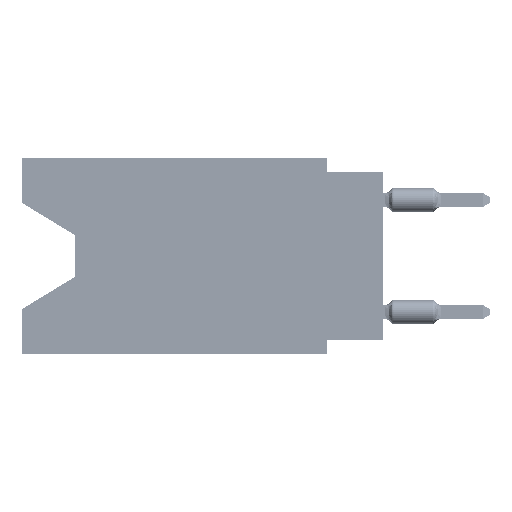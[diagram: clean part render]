
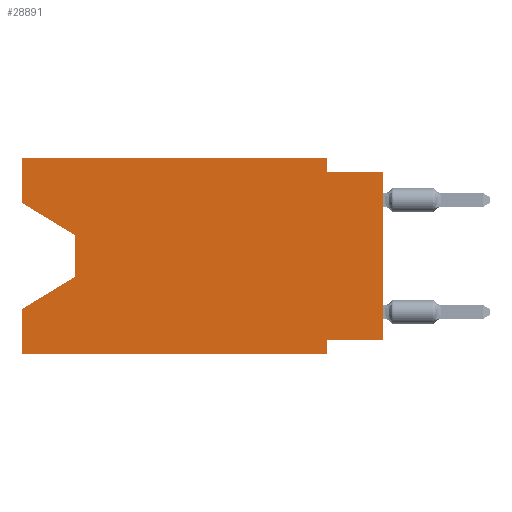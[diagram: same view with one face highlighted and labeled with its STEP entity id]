
A CAD part, left-side view. The second image highlights one B-rep face of the part: STEP entity #28891.
In plain terms, the highlighted planar face has unit normal (-1, 0, 0).
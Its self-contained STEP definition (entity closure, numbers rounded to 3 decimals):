
#560 = CARTESIAN_POINT ( 'NONE',  ( 0., 16.383, -6.852 ) ) ;
#1121 = ORIENTED_EDGE ( 'NONE', *, *, #41987, .T. ) ;
#3770 = VECTOR ( 'NONE', #63906, 1000. ) ;
#4355 = DIRECTION ( 'NONE',  ( 0., 1., 0. ) ) ;
#5054 = ORIENTED_EDGE ( 'NONE', *, *, #59475, .F. ) ;
#6071 = ORIENTED_EDGE ( 'NONE', *, *, #56471, .T. ) ;
#8778 = ORIENTED_EDGE ( 'NONE', *, *, #46111, .F. ) ;
#10045 = EDGE_CURVE ( 'NONE', #20409, #16009, #28303, .T. ) ;
#10096 = DIRECTION ( 'NONE',  ( 0., -1., 0. ) ) ;
#10343 = VECTOR ( 'NONE', #23110, 1000. ) ;
#10506 = ORIENTED_EDGE ( 'NONE', *, *, #18751, .T. ) ;
#11762 = VECTOR ( 'NONE', #4355, 1000. ) ;
#12016 = CARTESIAN_POINT ( 'NONE',  ( 0., 0., -8.255 ) ) ;
#12068 = CARTESIAN_POINT ( 'NONE',  ( 0., 16.383, -2.038 ) ) ;
#12527 = VERTEX_POINT ( 'NONE', #19864 ) ;
#12535 = CARTESIAN_POINT ( 'NONE',  ( 0., 16.383, -2.038 ) ) ;
#14194 = EDGE_CURVE ( 'NONE', #54865, #21545, #33069, .T. ) ;
#14480 = DIRECTION ( 'NONE',  ( 0., 0., 1. ) ) ;
#14519 = EDGE_CURVE ( 'NONE', #12527, #45243, #57657, .T. ) ;
#15418 = LINE ( 'NONE', #22644, #11762 ) ;
#16009 = VERTEX_POINT ( 'NONE', #64974 ) ;
#16568 = PLANE ( 'NONE',  #68132 ) ;
#17599 = DIRECTION ( 'NONE',  ( 0., 0., 1. ) ) ;
#18534 = CARTESIAN_POINT ( 'NONE',  ( 0., 16.383, 0. ) ) ;
#18751 = EDGE_CURVE ( 'NONE', #20409, #54865, #30435, .T. ) ;
#19864 = CARTESIAN_POINT ( 'NONE',  ( 0., 2.54, -0.635 ) ) ;
#20268 = CARTESIAN_POINT ( 'NONE',  ( 0., 16.383, -8.89 ) ) ;
#20409 = VERTEX_POINT ( 'NONE', #12068 ) ;
#21099 = VERTEX_POINT ( 'NONE', #33306 ) ;
#21545 = VERTEX_POINT ( 'NONE', #29250 ) ;
#21775 = ORIENTED_EDGE ( 'NONE', *, *, #10045, .F. ) ;
#22197 = DIRECTION ( 'NONE',  ( 0., -1., 0. ) ) ;
#22376 = CARTESIAN_POINT ( 'NONE',  ( 0., 13.97, -3.505 ) ) ;
#22507 = CARTESIAN_POINT ( 'NONE',  ( 0., 2.54, -8.89 ) ) ;
#22644 = CARTESIAN_POINT ( 'NONE',  ( 0., 0., -8.255 ) ) ;
#22863 = VECTOR ( 'NONE', #27706, 1000. ) ;
#23110 = DIRECTION ( 'NONE',  ( 0., 0., 1. ) ) ;
#23368 = DIRECTION ( 'NONE',  ( 0., 0.855, -0.519 ) ) ;
#24882 = LINE ( 'NONE', #20268, #63633 ) ;
#26849 = CARTESIAN_POINT ( 'NONE',  ( 0., 16.383, 0. ) ) ;
#27547 = CARTESIAN_POINT ( 'NONE',  ( 0., 16.383, -8.89 ) ) ;
#27696 = LINE ( 'NONE', #46357, #3770 ) ;
#27706 = DIRECTION ( 'NONE',  ( 0., 0., -1. ) ) ;
#28303 = LINE ( 'NONE', #29426, #34003 ) ;
#28891 = ADVANCED_FACE ( 'NONE', ( #69191 ), #16568, .F. ) ;
#29250 = CARTESIAN_POINT ( 'NONE',  ( 0., 13.97, -5.385 ) ) ;
#29426 = CARTESIAN_POINT ( 'NONE',  ( 0., 16.383, 0. ) ) ;
#30435 = LINE ( 'NONE', #12535, #47623 ) ;
#31227 = EDGE_CURVE ( 'NONE', #48847, #12527, #27696, .T. ) ;
#31349 = DIRECTION ( 'NONE',  ( 0., -1., 0. ) ) ;
#32784 = CARTESIAN_POINT ( 'NONE',  ( 0., 0., -0.635 ) ) ;
#33069 = LINE ( 'NONE', #22376, #22863 ) ;
#33306 = CARTESIAN_POINT ( 'NONE',  ( 0., 2.54, -8.89 ) ) ;
#33958 = ORIENTED_EDGE ( 'NONE', *, *, #34005, .T. ) ;
#34003 = VECTOR ( 'NONE', #17599, 1000. ) ;
#34005 = EDGE_CURVE ( 'NONE', #21545, #65468, #58437, .T. ) ;
#37012 = CARTESIAN_POINT ( 'NONE',  ( 0., 0., 0. ) ) ;
#38699 = DIRECTION ( 'NONE',  ( 0., 0., -1. ) ) ;
#41537 = VECTOR ( 'NONE', #69793, 1000. ) ;
#41711 = CARTESIAN_POINT ( 'NONE',  ( 0., 2.54, 0. ) ) ;
#41987 = EDGE_CURVE ( 'NONE', #45714, #45243, #66728, .T. ) ;
#42287 = CARTESIAN_POINT ( 'NONE',  ( 0., 2.54, -8.255 ) ) ;
#44096 = VECTOR ( 'NONE', #10096, 1000. ) ;
#44799 = VECTOR ( 'NONE', #22197, 1000. ) ;
#45243 = VERTEX_POINT ( 'NONE', #32784 ) ;
#45506 = CARTESIAN_POINT ( 'NONE',  ( 0., 13.97, -3.505 ) ) ;
#45714 = VERTEX_POINT ( 'NONE', #12016 ) ;
#46111 = EDGE_CURVE ( 'NONE', #16009, #48847, #55828, .T. ) ;
#46357 = CARTESIAN_POINT ( 'NONE',  ( 0., 2.54, 0. ) ) ;
#46625 = CARTESIAN_POINT ( 'NONE',  ( 0., 13.97, -5.385 ) ) ;
#47623 = VECTOR ( 'NONE', #59049, 1000. ) ;
#48847 = VERTEX_POINT ( 'NONE', #41711 ) ;
#49110 = VECTOR ( 'NONE', #23368, 1000. ) ;
#50377 = VERTEX_POINT ( 'NONE', #27547 ) ;
#51847 = LINE ( 'NONE', #22507, #41537 ) ;
#53421 = EDGE_CURVE ( 'NONE', #53521, #21099, #51847, .T. ) ;
#53521 = VERTEX_POINT ( 'NONE', #42287 ) ;
#54865 = VERTEX_POINT ( 'NONE', #45506 ) ;
#55828 = LINE ( 'NONE', #26849, #44096 ) ;
#56471 = EDGE_CURVE ( 'NONE', #50377, #21099, #24882, .T. ) ;
#57657 = LINE ( 'NONE', #74431, #44799 ) ;
#58437 = LINE ( 'NONE', #46625, #49110 ) ;
#58624 = ORIENTED_EDGE ( 'NONE', *, *, #14519, .F. ) ;
#59049 = DIRECTION ( 'NONE',  ( 0., -0.855, -0.519 ) ) ;
#59475 = EDGE_CURVE ( 'NONE', #50377, #65468, #63925, .T. ) ;
#60510 = ORIENTED_EDGE ( 'NONE', *, *, #72580, .F. ) ;
#63087 = DIRECTION ( 'NONE',  ( 1., 0., 0. ) ) ;
#63633 = VECTOR ( 'NONE', #31349, 1000. ) ;
#63906 = DIRECTION ( 'NONE',  ( 0., 0., -1. ) ) ;
#63925 = LINE ( 'NONE', #18534, #10343 ) ;
#63964 = ORIENTED_EDGE ( 'NONE', *, *, #31227, .F. ) ;
#64974 = CARTESIAN_POINT ( 'NONE',  ( 0., 16.383, 0. ) ) ;
#65468 = VERTEX_POINT ( 'NONE', #560 ) ;
#66728 = LINE ( 'NONE', #37012, #69541 ) ;
#68132 = AXIS2_PLACEMENT_3D ( 'NONE', #73771, #63087, #38699 ) ;
#69191 = FACE_OUTER_BOUND ( 'NONE', #74402, .T. ) ;
#69541 = VECTOR ( 'NONE', #14480, 1000. ) ;
#69793 = DIRECTION ( 'NONE',  ( 0., 0., -1. ) ) ;
#71229 = ORIENTED_EDGE ( 'NONE', *, *, #53421, .F. ) ;
#72580 = EDGE_CURVE ( 'NONE', #45714, #53521, #15418, .T. ) ;
#73542 = ORIENTED_EDGE ( 'NONE', *, *, #14194, .T. ) ;
#73771 = CARTESIAN_POINT ( 'NONE',  ( 0., 16.383, 0. ) ) ;
#74402 = EDGE_LOOP ( 'NONE', ( #10506, #73542, #33958, #5054, #6071, #71229, #60510, #1121, #58624, #63964, #8778, #21775 ) ) ;
#74431 = CARTESIAN_POINT ( 'NONE',  ( 0., 0., -0.635 ) ) ;
